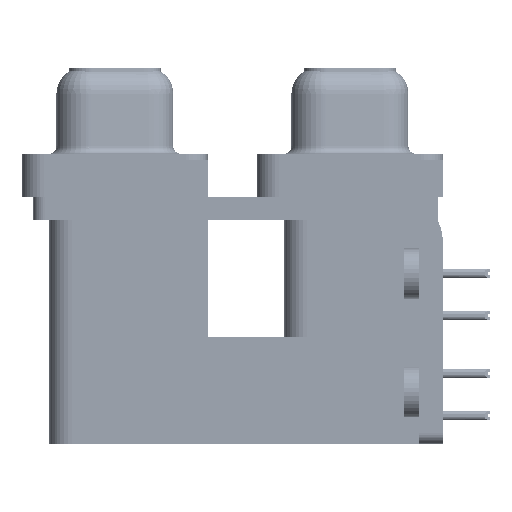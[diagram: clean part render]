
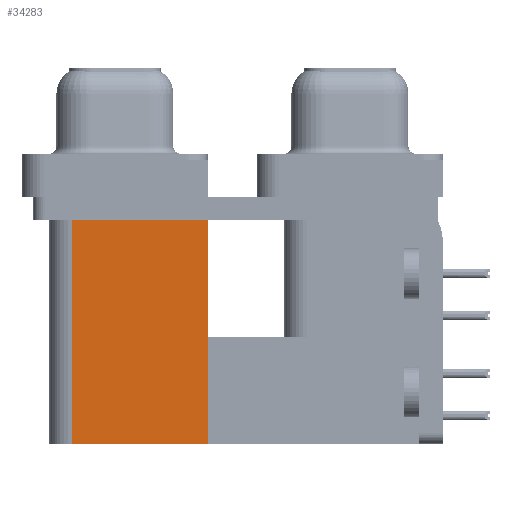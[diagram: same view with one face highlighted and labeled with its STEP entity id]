
A CAD part, left-side view. The second image highlights one B-rep face of the part: STEP entity #34283.
In plain terms, the highlighted planar face has unit normal (-1, 0, 0).
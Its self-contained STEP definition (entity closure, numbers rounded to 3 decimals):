
#1646 = LINE ( 'NONE', #21089, #12873 ) ;
#1785 = DIRECTION ( 'NONE',  ( 0., 1., 0. ) ) ;
#3248 = ORIENTED_EDGE ( 'NONE', *, *, #22656, .T. ) ;
#3595 = CARTESIAN_POINT ( 'NONE',  ( 3.7, 18.8, -2.5 ) ) ;
#5152 = CARTESIAN_POINT ( 'NONE',  ( 3.7, 9.6, -19.2 ) ) ;
#5962 = CARTESIAN_POINT ( 'NONE',  ( 3.7, 18.8, -19.2 ) ) ;
#6902 = DIRECTION ( 'NONE',  ( 1., 0., 0. ) ) ;
#9635 = LINE ( 'NONE', #51939, #37773 ) ;
#9801 = AXIS2_PLACEMENT_3D ( 'NONE', #25993, #6902, #1785 ) ;
#10736 = PLANE ( 'NONE',  #9801 ) ;
#12873 = VECTOR ( 'NONE', #36320, 1000. ) ;
#17578 = LINE ( 'NONE', #57002, #32884 ) ;
#18250 = DIRECTION ( 'NONE',  ( 0., 0., 1. ) ) ;
#21089 = CARTESIAN_POINT ( 'NONE',  ( 3.7, 18.8, -19.2 ) ) ;
#22656 = EDGE_CURVE ( 'NONE', #33863, #51473, #9635, .T. ) ;
#24064 = ORIENTED_EDGE ( 'NONE', *, *, #46602, .F. ) ;
#24574 = DIRECTION ( 'NONE',  ( 0., 1., 0. ) ) ;
#25993 = CARTESIAN_POINT ( 'NONE',  ( 3.7, 9.6, -19.2 ) ) ;
#27070 = EDGE_LOOP ( 'NONE', ( #60390, #52799, #24064, #3248 ) ) ;
#32884 = VECTOR ( 'NONE', #33445, 1000. ) ;
#33445 = DIRECTION ( 'NONE',  ( 0., 1., 0. ) ) ;
#33863 = VERTEX_POINT ( 'NONE', #47423 ) ;
#34220 = VERTEX_POINT ( 'NONE', #5962 ) ;
#34283 = ADVANCED_FACE ( 'NONE', ( #50132 ), #10736, .F. ) ;
#36231 = EDGE_CURVE ( 'NONE', #34220, #42108, #1646, .T. ) ;
#36320 = DIRECTION ( 'NONE',  ( 0., 0., 1. ) ) ;
#37773 = VECTOR ( 'NONE', #18250, 1000. ) ;
#41075 = EDGE_CURVE ( 'NONE', #51473, #42108, #17578, .T. ) ;
#42108 = VERTEX_POINT ( 'NONE', #3595 ) ;
#46602 = EDGE_CURVE ( 'NONE', #33863, #34220, #48715, .T. ) ;
#47423 = CARTESIAN_POINT ( 'NONE',  ( 3.7, 9.6, -19.2 ) ) ;
#48715 = LINE ( 'NONE', #5152, #55478 ) ;
#50132 = FACE_OUTER_BOUND ( 'NONE', #27070, .T. ) ;
#51473 = VERTEX_POINT ( 'NONE', #56951 ) ;
#51939 = CARTESIAN_POINT ( 'NONE',  ( 3.7, 9.6, -19.2 ) ) ;
#52799 = ORIENTED_EDGE ( 'NONE', *, *, #36231, .F. ) ;
#55478 = VECTOR ( 'NONE', #24574, 1000. ) ;
#56951 = CARTESIAN_POINT ( 'NONE',  ( 3.7, 9.6, -2.5 ) ) ;
#57002 = CARTESIAN_POINT ( 'NONE',  ( 3.7, 9.6, -2.5 ) ) ;
#60390 = ORIENTED_EDGE ( 'NONE', *, *, #41075, .T. ) ;
